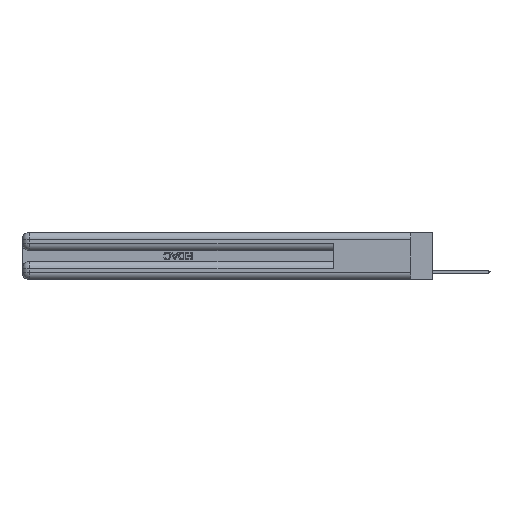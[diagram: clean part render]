
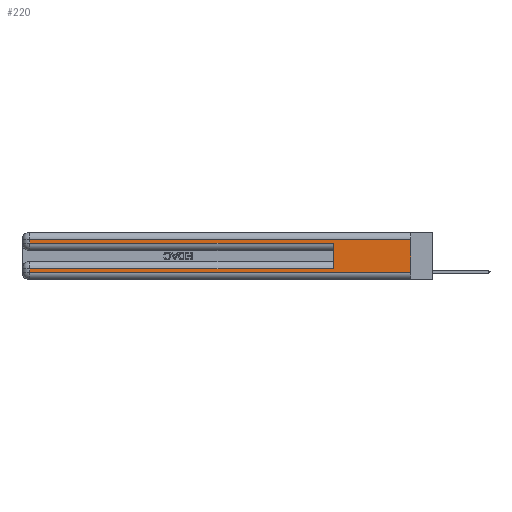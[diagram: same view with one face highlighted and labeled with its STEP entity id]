
A CAD part, left-side view. The second image highlights one B-rep face of the part: STEP entity #220.
In plain terms, the highlighted planar face has unit normal (-1, 0, 0).
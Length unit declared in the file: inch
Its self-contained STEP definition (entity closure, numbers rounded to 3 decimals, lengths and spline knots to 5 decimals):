
#50 = EDGE_CURVE ( 'NONE', #22299, #13642, #26868, .T. ) ;
#220 = ADVANCED_FACE ( 'NONE', ( #9336 ), #13230, .F. ) ;
#298 = VERTEX_POINT ( 'NONE', #1711 ) ;
#793 = LINE ( 'NONE', #12554, #27309 ) ;
#1711 = CARTESIAN_POINT ( 'NONE',  ( 0., 2.94, 0.31 ) ) ;
#2020 = CARTESIAN_POINT ( 'NONE',  ( 0., 2.94, 0.37 ) ) ;
#2550 = VECTOR ( 'NONE', #21696, 39.37008 ) ;
#2612 = CARTESIAN_POINT ( 'NONE',  ( 0., 2.94, 0.285 ) ) ;
#2673 = CARTESIAN_POINT ( 'NONE',  ( 0., 0., 0.37 ) ) ;
#2813 = CARTESIAN_POINT ( 'NONE',  ( 0., 2.94, 0.06 ) ) ;
#3027 = CARTESIAN_POINT ( 'NONE',  ( 0., 0., 0.085 ) ) ;
#3235 = CARTESIAN_POINT ( 'NONE',  ( 0., 0.6, 0.085 ) ) ;
#3522 = EDGE_CURVE ( 'NONE', #17468, #17321, #15940, .T. ) ;
#3727 = CARTESIAN_POINT ( 'NONE',  ( 0., 0., 0.06 ) ) ;
#4212 = DIRECTION ( 'NONE',  ( 0., 1., 0. ) ) ;
#4264 = AXIS2_PLACEMENT_3D ( 'NONE', #21389, #11387, #23888 ) ;
#4305 = ORIENTED_EDGE ( 'NONE', *, *, #19235, .T. ) ;
#5433 = EDGE_CURVE ( 'NONE', #22299, #298, #6484, .T. ) ;
#6084 = EDGE_CURVE ( 'NONE', #298, #22562, #18546, .T. ) ;
#6484 = LINE ( 'NONE', #24141, #14265 ) ;
#6742 = LINE ( 'NONE', #3727, #10680 ) ;
#6852 = LINE ( 'NONE', #29282, #2550 ) ;
#8127 = CARTESIAN_POINT ( 'NONE',  ( 0., 0., 0.31 ) ) ;
#8170 = ORIENTED_EDGE ( 'NONE', *, *, #3522, .T. ) ;
#8339 = EDGE_CURVE ( 'NONE', #17468, #30921, #793, .T. ) ;
#9336 = FACE_OUTER_BOUND ( 'NONE', #23798, .T. ) ;
#9786 = EDGE_CURVE ( 'NONE', #19041, #13642, #6742, .T. ) ;
#10349 = VECTOR ( 'NONE', #24271, 39.37008 ) ;
#10680 = VECTOR ( 'NONE', #31393, 39.37008 ) ;
#11387 = DIRECTION ( 'NONE',  ( 1., 0., 0. ) ) ;
#12512 = DIRECTION ( 'NONE',  ( 0., -1., 0. ) ) ;
#12554 = CARTESIAN_POINT ( 'NONE',  ( 0., 0.6, 0.145 ) ) ;
#13230 = PLANE ( 'NONE',  #4264 ) ;
#13642 = VERTEX_POINT ( 'NONE', #24063 ) ;
#14265 = VECTOR ( 'NONE', #4212, 39.37008 ) ;
#15512 = ORIENTED_EDGE ( 'NONE', *, *, #6084, .T. ) ;
#15940 = LINE ( 'NONE', #3027, #17508 ) ;
#16525 = VECTOR ( 'NONE', #12512, 39.37008 ) ;
#16584 = ORIENTED_EDGE ( 'NONE', *, *, #9786, .T. ) ;
#17321 = VERTEX_POINT ( 'NONE', #31260 ) ;
#17468 = VERTEX_POINT ( 'NONE', #3235 ) ;
#17508 = VECTOR ( 'NONE', #27867, 39.37008 ) ;
#17642 = DIRECTION ( 'NONE',  ( 0., 0., -1. ) ) ;
#18546 = LINE ( 'NONE', #2020, #10349 ) ;
#19041 = VERTEX_POINT ( 'NONE', #2813 ) ;
#19235 = EDGE_CURVE ( 'NONE', #17321, #19041, #6852, .T. ) ;
#21250 = ORIENTED_EDGE ( 'NONE', *, *, #5433, .T. ) ;
#21389 = CARTESIAN_POINT ( 'NONE',  ( 0., 0., 0.37 ) ) ;
#21696 = DIRECTION ( 'NONE',  ( 0., 0., -1. ) ) ;
#21950 = CARTESIAN_POINT ( 'NONE',  ( 0., 0.6, 0.285 ) ) ;
#22299 = VERTEX_POINT ( 'NONE', #8127 ) ;
#22562 = VERTEX_POINT ( 'NONE', #2612 ) ;
#22655 = ORIENTED_EDGE ( 'NONE', *, *, #8339, .F. ) ;
#23165 = ORIENTED_EDGE ( 'NONE', *, *, #26398, .T. ) ;
#23798 = EDGE_LOOP ( 'NONE', ( #28189, #21250, #15512, #23165, #22655, #8170, #4305, #16584 ) ) ;
#23888 = DIRECTION ( 'NONE',  ( 0., 0., -1. ) ) ;
#24063 = CARTESIAN_POINT ( 'NONE',  ( 0., 0., 0.06 ) ) ;
#24141 = CARTESIAN_POINT ( 'NONE',  ( 0., 0., 0.31 ) ) ;
#24271 = DIRECTION ( 'NONE',  ( 0., 0., -1. ) ) ;
#24997 = CARTESIAN_POINT ( 'NONE',  ( 0., 0., 0.285 ) ) ;
#25319 = VECTOR ( 'NONE', #17642, 39.37008 ) ;
#26398 = EDGE_CURVE ( 'NONE', #22562, #30921, #31323, .T. ) ;
#26868 = LINE ( 'NONE', #2673, #25319 ) ;
#27309 = VECTOR ( 'NONE', #29736, 39.37008 ) ;
#27867 = DIRECTION ( 'NONE',  ( 0., 1., 0. ) ) ;
#28189 = ORIENTED_EDGE ( 'NONE', *, *, #50, .F. ) ;
#29282 = CARTESIAN_POINT ( 'NONE',  ( 0., 2.94, 0.37 ) ) ;
#29736 = DIRECTION ( 'NONE',  ( 0., 0., 1. ) ) ;
#30921 = VERTEX_POINT ( 'NONE', #21950 ) ;
#31260 = CARTESIAN_POINT ( 'NONE',  ( 0., 2.94, 0.085 ) ) ;
#31323 = LINE ( 'NONE', #24997, #16525 ) ;
#31393 = DIRECTION ( 'NONE',  ( 0., -1., 0. ) ) ;
